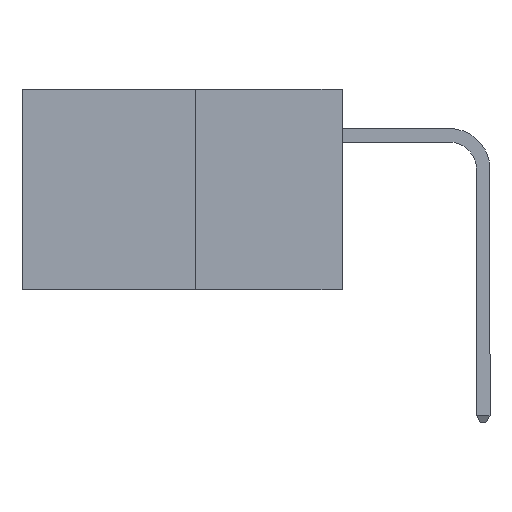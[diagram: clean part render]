
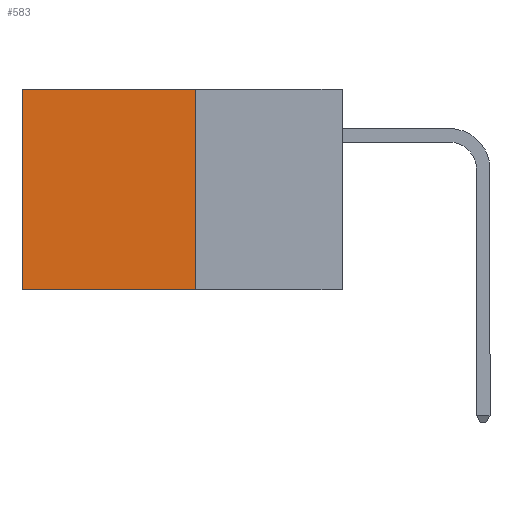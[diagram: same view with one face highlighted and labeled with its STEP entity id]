
A CAD part, left-side view. The second image highlights one B-rep face of the part: STEP entity #583.
In plain terms, the highlighted planar face has unit normal (-1, 0, 0).
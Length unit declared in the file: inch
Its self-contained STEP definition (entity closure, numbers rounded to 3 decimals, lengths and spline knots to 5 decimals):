
#583 = ADVANCED_FACE ( 'NONE', ( #28962 ), #9616, .F. ) ;
#1022 = EDGE_CURVE ( 'NONE', #19345, #16606, #22487, .T. ) ;
#1339 = AXIS2_PLACEMENT_3D ( 'NONE', #6465, #16822, #19586 ) ;
#1615 = CARTESIAN_POINT ( 'NONE',  ( 0.277, 0.27, -0.37 ) ) ;
#1659 = VECTOR ( 'NONE', #22133, 39.37008 ) ;
#3406 = DIRECTION ( 'NONE',  ( 0., 0., -1. ) ) ;
#5081 = VERTEX_POINT ( 'NONE', #8058 ) ;
#5192 = ORIENTED_EDGE ( 'NONE', *, *, #17032, .F. ) ;
#5616 = DIRECTION ( 'NONE',  ( 0., 1., 0. ) ) ;
#6465 = CARTESIAN_POINT ( 'NONE',  ( 0.277, 0.27, -0.37 ) ) ;
#8058 = CARTESIAN_POINT ( 'NONE',  ( 0.277, 0.27, 0. ) ) ;
#9343 = LINE ( 'NONE', #1615, #14086 ) ;
#9616 = PLANE ( 'NONE',  #1339 ) ;
#11345 = CARTESIAN_POINT ( 'NONE',  ( 0.277, 0.27, -0.37 ) ) ;
#11527 = ORIENTED_EDGE ( 'NONE', *, *, #24422, .T. ) ;
#12290 = CARTESIAN_POINT ( 'NONE',  ( 0.277, 0.59, -0.37 ) ) ;
#13146 = LINE ( 'NONE', #19578, #13878 ) ;
#13857 = ORIENTED_EDGE ( 'NONE', *, *, #1022, .T. ) ;
#13878 = VECTOR ( 'NONE', #5616, 39.37008 ) ;
#14086 = VECTOR ( 'NONE', #15984, 39.37008 ) ;
#15012 = EDGE_LOOP ( 'NONE', ( #13857, #15692, #5192, #11527 ) ) ;
#15692 = ORIENTED_EDGE ( 'NONE', *, *, #16194, .F. ) ;
#15984 = DIRECTION ( 'NONE',  ( 0., 0., -1. ) ) ;
#16194 = EDGE_CURVE ( 'NONE', #18982, #16606, #20550, .T. ) ;
#16606 = VERTEX_POINT ( 'NONE', #12290 ) ;
#16822 = DIRECTION ( 'NONE',  ( 1., 0., 0. ) ) ;
#17032 = EDGE_CURVE ( 'NONE', #5081, #18982, #9343, .T. ) ;
#17950 = CARTESIAN_POINT ( 'NONE',  ( 0.277, 0.59, -0.37 ) ) ;
#18982 = VERTEX_POINT ( 'NONE', #11345 ) ;
#19345 = VERTEX_POINT ( 'NONE', #24171 ) ;
#19578 = CARTESIAN_POINT ( 'NONE',  ( 0.277, 0.27, 0. ) ) ;
#19586 = DIRECTION ( 'NONE',  ( 0., 0., -1. ) ) ;
#20550 = LINE ( 'NONE', #24346, #1659 ) ;
#22133 = DIRECTION ( 'NONE',  ( 0., 1., 0. ) ) ;
#22487 = LINE ( 'NONE', #17950, #27850 ) ;
#24171 = CARTESIAN_POINT ( 'NONE',  ( 0.277, 0.59, 0. ) ) ;
#24346 = CARTESIAN_POINT ( 'NONE',  ( 0.277, 0.27, -0.37 ) ) ;
#24422 = EDGE_CURVE ( 'NONE', #5081, #19345, #13146, .T. ) ;
#27850 = VECTOR ( 'NONE', #3406, 39.37008 ) ;
#28962 = FACE_OUTER_BOUND ( 'NONE', #15012, .T. ) ;
